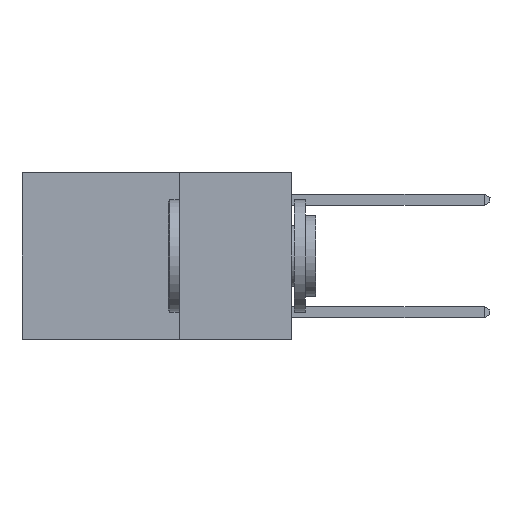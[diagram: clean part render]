
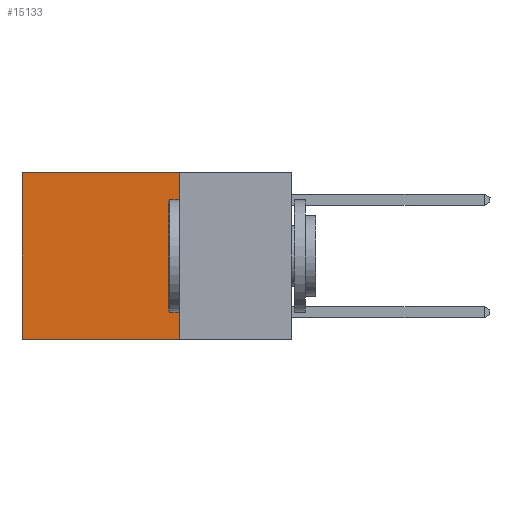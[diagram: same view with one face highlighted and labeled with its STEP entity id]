
A CAD part, left-side view. The second image highlights one B-rep face of the part: STEP entity #15133.
In plain terms, the highlighted planar face has unit normal (-1, 0, 0).
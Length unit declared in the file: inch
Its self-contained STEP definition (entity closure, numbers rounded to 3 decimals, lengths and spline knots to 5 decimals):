
#485 = AXIS2_PLACEMENT_3D ( 'NONE', #2099, #8016, #13941 ) ;
#550 = LINE ( 'NONE', #6468, #8800 ) ;
#734 = EDGE_CURVE ( 'NONE', #5176, #11978, #16403, .T. ) ;
#1768 = VERTEX_POINT ( 'NONE', #18093 ) ;
#1858 = VECTOR ( 'NONE', #2871, 39.37008 ) ;
#1862 = DIRECTION ( 'NONE',  ( 0., 1., 0. ) ) ;
#2099 = CARTESIAN_POINT ( 'NONE',  ( 0.2625, 0.25, 0. ) ) ;
#2871 = DIRECTION ( 'NONE',  ( 0., 0., -1. ) ) ;
#3064 = CARTESIAN_POINT ( 'NONE',  ( 0.2625, 0.25, 0. ) ) ;
#5014 = DIRECTION ( 'NONE',  ( 0., 0., -1. ) ) ;
#5176 = VERTEX_POINT ( 'NONE', #7688 ) ;
#6468 = CARTESIAN_POINT ( 'NONE',  ( 0.2625, 0.6, 0. ) ) ;
#6892 = VECTOR ( 'NONE', #15273, 39.37008 ) ;
#7688 = CARTESIAN_POINT ( 'NONE',  ( 0.2625, 0.25, 0. ) ) ;
#8012 = ORIENTED_EDGE ( 'NONE', *, *, #17835, .F. ) ;
#8016 = DIRECTION ( 'NONE',  ( 1., 0., 0. ) ) ;
#8025 = CARTESIAN_POINT ( 'NONE',  ( 0.2625, 0.25, -0.37 ) ) ;
#8800 = VECTOR ( 'NONE', #5014, 39.37008 ) ;
#9236 = LINE ( 'NONE', #13614, #6892 ) ;
#9248 = CARTESIAN_POINT ( 'NONE',  ( 0.2625, 0.25, -0.37 ) ) ;
#9283 = FACE_OUTER_BOUND ( 'NONE', #10036, .T. ) ;
#9422 = VERTEX_POINT ( 'NONE', #14413 ) ;
#10036 = EDGE_LOOP ( 'NONE', ( #19052, #8012, #11149, #11164 ) ) ;
#11149 = ORIENTED_EDGE ( 'NONE', *, *, #734, .F. ) ;
#11164 = ORIENTED_EDGE ( 'NONE', *, *, #11391, .T. ) ;
#11391 = EDGE_CURVE ( 'NONE', #5176, #1768, #9236, .T. ) ;
#11978 = VERTEX_POINT ( 'NONE', #8025 ) ;
#13614 = CARTESIAN_POINT ( 'NONE',  ( 0.2625, 0.25, 0. ) ) ;
#13941 = DIRECTION ( 'NONE',  ( 0., 0., -1. ) ) ;
#14413 = CARTESIAN_POINT ( 'NONE',  ( 0.2625, 0.6, -0.37 ) ) ;
#15133 = ADVANCED_FACE ( 'NONE', ( #9283 ), #18335, .F. ) ;
#15273 = DIRECTION ( 'NONE',  ( 0., 1., 0. ) ) ;
#16403 = LINE ( 'NONE', #3064, #1858 ) ;
#16666 = LINE ( 'NONE', #9248, #18157 ) ;
#16904 = EDGE_CURVE ( 'NONE', #1768, #9422, #550, .T. ) ;
#17835 = EDGE_CURVE ( 'NONE', #11978, #9422, #16666, .T. ) ;
#18093 = CARTESIAN_POINT ( 'NONE',  ( 0.2625, 0.6, 0. ) ) ;
#18157 = VECTOR ( 'NONE', #1862, 39.37008 ) ;
#18335 = PLANE ( 'NONE',  #485 ) ;
#19052 = ORIENTED_EDGE ( 'NONE', *, *, #16904, .T. ) ;
